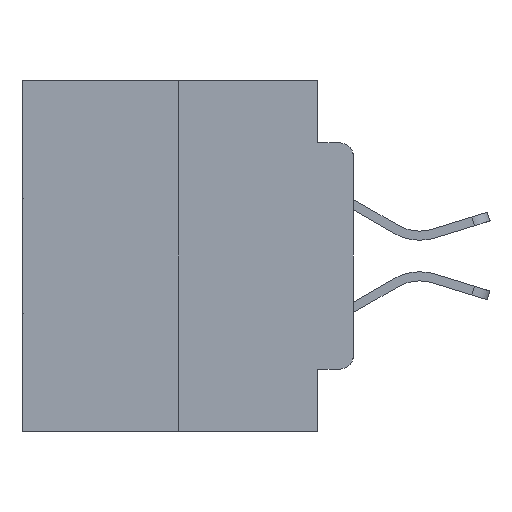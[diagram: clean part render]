
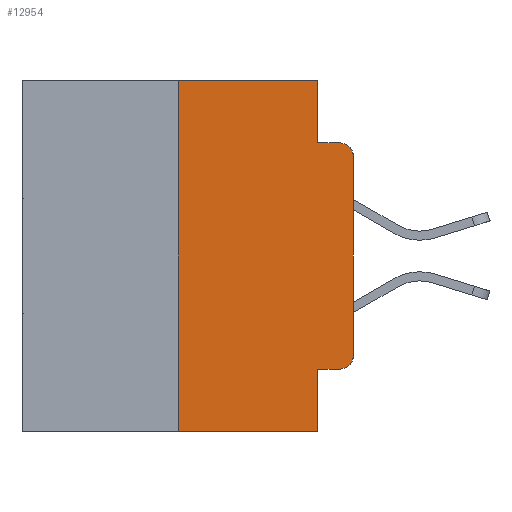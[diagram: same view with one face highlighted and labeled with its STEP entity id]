
A CAD part, left-side view. The second image highlights one B-rep face of the part: STEP entity #12954.
In plain terms, the highlighted planar face has unit normal (-1, 0, 0).
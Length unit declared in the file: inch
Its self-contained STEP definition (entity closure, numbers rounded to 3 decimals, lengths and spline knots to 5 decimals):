
#35 = DIRECTION ( 'NONE',  ( 0., 0., -1. ) ) ;
#349 = VECTOR ( 'NONE', #3812, 39.37008 ) ;
#618 = VERTEX_POINT ( 'NONE', #6938 ) ;
#1489 = DIRECTION ( 'NONE',  ( 0., 0., -1. ) ) ;
#1506 = EDGE_CURVE ( 'NONE', #26441, #1636, #2596, .T. ) ;
#1636 = VERTEX_POINT ( 'NONE', #18137 ) ;
#2596 = LINE ( 'NONE', #18536, #24756 ) ;
#3039 = EDGE_CURVE ( 'NONE', #13240, #9253, #23380, .T. ) ;
#3041 = CARTESIAN_POINT ( 'NONE',  ( 0., 0.25, -0.5 ) ) ;
#3197 = ORIENTED_EDGE ( 'NONE', *, *, #1506, .F. ) ;
#3579 = VERTEX_POINT ( 'NONE', #25440 ) ;
#3812 = DIRECTION ( 'NONE',  ( 0., 0., 1. ) ) ;
#4872 = ORIENTED_EDGE ( 'NONE', *, *, #11467, .T. ) ;
#4886 = VECTOR ( 'NONE', #24527, 39.37008 ) ;
#5137 = EDGE_CURVE ( 'NONE', #9253, #23045, #14213, .T. ) ;
#5457 = VECTOR ( 'NONE', #7361, 39.37008 ) ;
#5585 = LINE ( 'NONE', #14170, #4886 ) ;
#6844 = CARTESIAN_POINT ( 'NONE',  ( 0., 0.051, 0. ) ) ;
#6938 = CARTESIAN_POINT ( 'NONE',  ( 0., 0.02, -0.4115 ) ) ;
#7361 = DIRECTION ( 'NONE',  ( 0., -1., 0. ) ) ;
#7485 = CARTESIAN_POINT ( 'NONE',  ( 0., 0.051, -0.4115 ) ) ;
#7513 = CARTESIAN_POINT ( 'NONE',  ( 0., 0.051, -0.0885 ) ) ;
#8448 = VECTOR ( 'NONE', #16722, 39.37008 ) ;
#9253 = VERTEX_POINT ( 'NONE', #11320 ) ;
#10152 = ORIENTED_EDGE ( 'NONE', *, *, #23728, .T. ) ;
#10318 = EDGE_LOOP ( 'NONE', ( #4872, #18114, #18162, #26819, #10524, #19461, #14935, #3197, #26590, #10152 ) ) ;
#10423 = DIRECTION ( 'NONE',  ( 0., -1., 0. ) ) ;
#10524 = ORIENTED_EDGE ( 'NONE', *, *, #5137, .F. ) ;
#10773 = CARTESIAN_POINT ( 'NONE',  ( 0., 0., -0.3915 ) ) ;
#10985 = PLANE ( 'NONE',  #23049 ) ;
#11320 = CARTESIAN_POINT ( 'NONE',  ( 0., 0.25, 0. ) ) ;
#11467 = EDGE_CURVE ( 'NONE', #11752, #24416, #5585, .T. ) ;
#11699 = CARTESIAN_POINT ( 'NONE',  ( 0., 0.02, -0.1085 ) ) ;
#11752 = VERTEX_POINT ( 'NONE', #10773 ) ;
#11767 = LINE ( 'NONE', #22998, #22887 ) ;
#12954 = ADVANCED_FACE ( 'NONE', ( #24167 ), #10985, .F. ) ;
#13057 = CIRCLE ( 'NONE', #24775, 0.02 ) ;
#13140 = DIRECTION ( 'NONE',  ( 0., 0., -1. ) ) ;
#13240 = VERTEX_POINT ( 'NONE', #3041 ) ;
#13689 = CIRCLE ( 'NONE', #21879, 0.02 ) ;
#13862 = DIRECTION ( 'NONE',  ( 0., 0., -1. ) ) ;
#14072 = DIRECTION ( 'NONE',  ( 0., -1., 0. ) ) ;
#14170 = CARTESIAN_POINT ( 'NONE',  ( 0., 0., 0. ) ) ;
#14213 = LINE ( 'NONE', #22069, #8448 ) ;
#14390 = EDGE_CURVE ( 'NONE', #13240, #1636, #17012, .T. ) ;
#14511 = VECTOR ( 'NONE', #14072, 39.37008 ) ;
#14756 = DIRECTION ( 'NONE',  ( -1., 0., 0. ) ) ;
#14868 = EDGE_CURVE ( 'NONE', #23045, #3579, #22716, .T. ) ;
#14935 = ORIENTED_EDGE ( 'NONE', *, *, #14390, .T. ) ;
#15873 = LINE ( 'NONE', #7513, #14511 ) ;
#16196 = CARTESIAN_POINT ( 'NONE',  ( 0., 0.051, 0. ) ) ;
#16299 = EDGE_CURVE ( 'NONE', #3579, #25590, #15873, .T. ) ;
#16722 = DIRECTION ( 'NONE',  ( 0., -1., 0. ) ) ;
#17012 = LINE ( 'NONE', #26356, #5457 ) ;
#17226 = VECTOR ( 'NONE', #35, 39.37008 ) ;
#17997 = DIRECTION ( 'NONE',  ( 0., 0., -1. ) ) ;
#18114 = ORIENTED_EDGE ( 'NONE', *, *, #24607, .T. ) ;
#18137 = CARTESIAN_POINT ( 'NONE',  ( 0., 0.051, -0.5 ) ) ;
#18162 = ORIENTED_EDGE ( 'NONE', *, *, #16299, .F. ) ;
#18536 = CARTESIAN_POINT ( 'NONE',  ( 0., 0.051, 0. ) ) ;
#19461 = ORIENTED_EDGE ( 'NONE', *, *, #3039, .F. ) ;
#19560 = CARTESIAN_POINT ( 'NONE',  ( 0., 0., -0.1085 ) ) ;
#21576 = CARTESIAN_POINT ( 'NONE',  ( 0., 0.02, -0.0885 ) ) ;
#21879 = AXIS2_PLACEMENT_3D ( 'NONE', #11699, #26287, #13862 ) ;
#22069 = CARTESIAN_POINT ( 'NONE',  ( 0., 0.473, 0. ) ) ;
#22716 = LINE ( 'NONE', #6844, #17226 ) ;
#22887 = VECTOR ( 'NONE', #10423, 39.37008 ) ;
#22998 = CARTESIAN_POINT ( 'NONE',  ( 0., 0.051, -0.4115 ) ) ;
#23045 = VERTEX_POINT ( 'NONE', #16196 ) ;
#23049 = AXIS2_PLACEMENT_3D ( 'NONE', #23442, #25596, #13140 ) ;
#23380 = LINE ( 'NONE', #26135, #349 ) ;
#23442 = CARTESIAN_POINT ( 'NONE',  ( 0., 0.473, 0. ) ) ;
#23728 = EDGE_CURVE ( 'NONE', #618, #11752, #13057, .T. ) ;
#24167 = FACE_OUTER_BOUND ( 'NONE', #10318, .T. ) ;
#24416 = VERTEX_POINT ( 'NONE', #19560 ) ;
#24527 = DIRECTION ( 'NONE',  ( 0., 0., 1. ) ) ;
#24607 = EDGE_CURVE ( 'NONE', #24416, #25590, #13689, .T. ) ;
#24756 = VECTOR ( 'NONE', #17997, 39.37008 ) ;
#24775 = AXIS2_PLACEMENT_3D ( 'NONE', #27165, #14756, #1489 ) ;
#25440 = CARTESIAN_POINT ( 'NONE',  ( 0., 0.051, -0.0885 ) ) ;
#25590 = VERTEX_POINT ( 'NONE', #21576 ) ;
#25596 = DIRECTION ( 'NONE',  ( 1., 0., 0. ) ) ;
#26135 = CARTESIAN_POINT ( 'NONE',  ( 0., 0.25, 0. ) ) ;
#26287 = DIRECTION ( 'NONE',  ( -1., 0., 0. ) ) ;
#26356 = CARTESIAN_POINT ( 'NONE',  ( 0., 0.473, -0.5 ) ) ;
#26441 = VERTEX_POINT ( 'NONE', #7485 ) ;
#26590 = ORIENTED_EDGE ( 'NONE', *, *, #27207, .T. ) ;
#26819 = ORIENTED_EDGE ( 'NONE', *, *, #14868, .F. ) ;
#27165 = CARTESIAN_POINT ( 'NONE',  ( 0., 0.02, -0.3915 ) ) ;
#27207 = EDGE_CURVE ( 'NONE', #26441, #618, #11767, .T. ) ;
